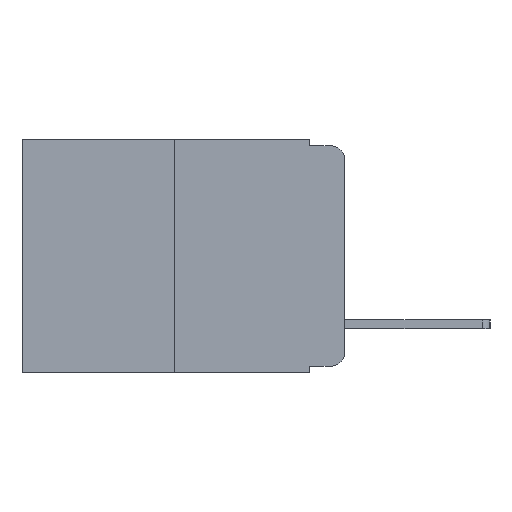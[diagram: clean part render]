
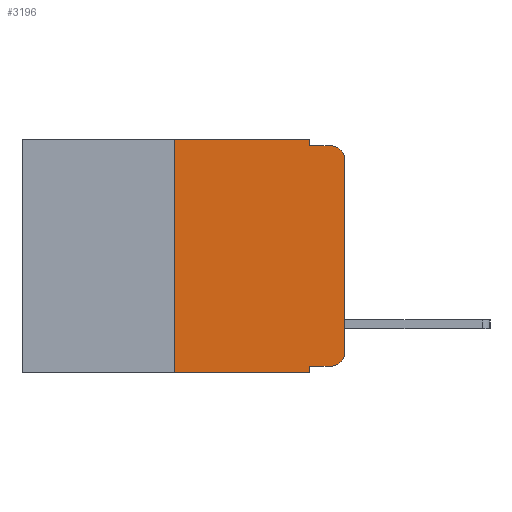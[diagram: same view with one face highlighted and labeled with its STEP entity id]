
A CAD part, left-side view. The second image highlights one B-rep face of the part: STEP entity #3196.
In plain terms, the highlighted planar face has unit normal (-1, 0, 0).
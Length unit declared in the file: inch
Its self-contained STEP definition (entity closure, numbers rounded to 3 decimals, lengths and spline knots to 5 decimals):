
#322 = EDGE_CURVE ( 'NONE', #18513, #15557, #9251, .T. ) ;
#994 = DIRECTION ( 'NONE',  ( 0., 0., 1. ) ) ;
#1172 = LINE ( 'NONE', #19652, #9362 ) ;
#1201 = ORIENTED_EDGE ( 'NONE', *, *, #19016, .F. ) ;
#1888 = DIRECTION ( 'NONE',  ( -1., 0., 0. ) ) ;
#2689 = CARTESIAN_POINT ( 'NONE',  ( 0., 0.051, -0.01 ) ) ;
#3196 = ADVANCED_FACE ( 'NONE', ( #18753 ), #17368, .F. ) ;
#3283 = ORIENTED_EDGE ( 'NONE', *, *, #15947, .F. ) ;
#3398 = VECTOR ( 'NONE', #13719, 39.37008 ) ;
#3613 = VECTOR ( 'NONE', #11609, 39.37008 ) ;
#3761 = VERTEX_POINT ( 'NONE', #12623 ) ;
#4547 = VERTEX_POINT ( 'NONE', #5112 ) ;
#4727 = LINE ( 'NONE', #5884, #12788 ) ;
#4770 = DIRECTION ( 'NONE',  ( 0., -1., 0. ) ) ;
#4900 = VERTEX_POINT ( 'NONE', #15831 ) ;
#5112 = CARTESIAN_POINT ( 'NONE',  ( 0., 0.25, -0.343 ) ) ;
#5862 = DIRECTION ( 'NONE',  ( 0., 0., -1. ) ) ;
#5884 = CARTESIAN_POINT ( 'NONE',  ( 0., 0., 0. ) ) ;
#6059 = CARTESIAN_POINT ( 'NONE',  ( 0., 0., -0.03 ) ) ;
#6288 = AXIS2_PLACEMENT_3D ( 'NONE', #11614, #1888, #13182 ) ;
#6341 = ORIENTED_EDGE ( 'NONE', *, *, #16486, .F. ) ;
#6467 = VERTEX_POINT ( 'NONE', #6059 ) ;
#6579 = CIRCLE ( 'NONE', #6288, 0.02 ) ;
#7234 = EDGE_CURVE ( 'NONE', #6467, #20227, #6579, .T. ) ;
#7325 = CARTESIAN_POINT ( 'NONE',  ( 0., 0.02, -0.313 ) ) ;
#7395 = EDGE_CURVE ( 'NONE', #20671, #7611, #10112, .T. ) ;
#7611 = VERTEX_POINT ( 'NONE', #8012 ) ;
#7755 = LINE ( 'NONE', #10516, #3398 ) ;
#7874 = DIRECTION ( 'NONE',  ( 1., 0., 0. ) ) ;
#8012 = CARTESIAN_POINT ( 'NONE',  ( 0., 0., -0.313 ) ) ;
#8069 = CARTESIAN_POINT ( 'NONE',  ( 0., 0.051, -0.333 ) ) ;
#8152 = ORIENTED_EDGE ( 'NONE', *, *, #10626, .T. ) ;
#8194 = EDGE_CURVE ( 'NONE', #4547, #3761, #9569, .T. ) ;
#8462 = LINE ( 'NONE', #9990, #3613 ) ;
#8744 = VECTOR ( 'NONE', #5862, 39.37008 ) ;
#8929 = DIRECTION ( 'NONE',  ( 0., 0., -1. ) ) ;
#9251 = LINE ( 'NONE', #17713, #8744 ) ;
#9362 = VECTOR ( 'NONE', #13468, 39.37008 ) ;
#9569 = LINE ( 'NONE', #17538, #17484 ) ;
#9679 = DIRECTION ( 'NONE',  ( 0., -1., 0. ) ) ;
#9990 = CARTESIAN_POINT ( 'NONE',  ( 0., 0.051, 0. ) ) ;
#10112 = CIRCLE ( 'NONE', #16995, 0.02 ) ;
#10162 = DIRECTION ( 'NONE',  ( 0., -1., 0. ) ) ;
#10207 = EDGE_LOOP ( 'NONE', ( #18019, #14394, #6341, #19964, #13643, #1201, #10905, #3283, #8152, #20697 ) ) ;
#10516 = CARTESIAN_POINT ( 'NONE',  ( 0., 0.473, 0. ) ) ;
#10626 = EDGE_CURVE ( 'NONE', #14865, #20671, #11202, .T. ) ;
#10905 = ORIENTED_EDGE ( 'NONE', *, *, #8194, .T. ) ;
#11202 = LINE ( 'NONE', #8069, #19018 ) ;
#11209 = VECTOR ( 'NONE', #10162, 39.37008 ) ;
#11609 = DIRECTION ( 'NONE',  ( 0., 0., -1. ) ) ;
#11614 = CARTESIAN_POINT ( 'NONE',  ( 0., 0.02, -0.03 ) ) ;
#12084 = EDGE_CURVE ( 'NONE', #4900, #18513, #7755, .T. ) ;
#12135 = CARTESIAN_POINT ( 'NONE',  ( 0., 0.051, -0.333 ) ) ;
#12215 = LINE ( 'NONE', #13364, #11209 ) ;
#12256 = CARTESIAN_POINT ( 'NONE',  ( 0., 0.051, 0. ) ) ;
#12623 = CARTESIAN_POINT ( 'NONE',  ( 0., 0.051, -0.343 ) ) ;
#12788 = VECTOR ( 'NONE', #994, 39.37008 ) ;
#13182 = DIRECTION ( 'NONE',  ( 0., 0., -1. ) ) ;
#13364 = CARTESIAN_POINT ( 'NONE',  ( 0., 0.051, -0.01 ) ) ;
#13468 = DIRECTION ( 'NONE',  ( 0., 0., 1. ) ) ;
#13643 = ORIENTED_EDGE ( 'NONE', *, *, #12084, .F. ) ;
#13719 = DIRECTION ( 'NONE',  ( 0., -1., 0. ) ) ;
#14394 = ORIENTED_EDGE ( 'NONE', *, *, #7234, .T. ) ;
#14865 = VERTEX_POINT ( 'NONE', #12135 ) ;
#15509 = CARTESIAN_POINT ( 'NONE',  ( 0., 0.02, -0.333 ) ) ;
#15557 = VERTEX_POINT ( 'NONE', #2689 ) ;
#15831 = CARTESIAN_POINT ( 'NONE',  ( 0., 0.25, 0. ) ) ;
#15947 = EDGE_CURVE ( 'NONE', #14865, #3761, #8462, .T. ) ;
#16486 = EDGE_CURVE ( 'NONE', #15557, #20227, #12215, .T. ) ;
#16995 = AXIS2_PLACEMENT_3D ( 'NONE', #7325, #18377, #8929 ) ;
#17368 = PLANE ( 'NONE',  #17789 ) ;
#17484 = VECTOR ( 'NONE', #4770, 39.37008 ) ;
#17538 = CARTESIAN_POINT ( 'NONE',  ( 0., 0.473, -0.343 ) ) ;
#17664 = CARTESIAN_POINT ( 'NONE',  ( 0., 0.02, -0.01 ) ) ;
#17713 = CARTESIAN_POINT ( 'NONE',  ( 0., 0.051, 0. ) ) ;
#17789 = AXIS2_PLACEMENT_3D ( 'NONE', #20415, #7874, #18898 ) ;
#18019 = ORIENTED_EDGE ( 'NONE', *, *, #20690, .T. ) ;
#18377 = DIRECTION ( 'NONE',  ( -1., 0., 0. ) ) ;
#18513 = VERTEX_POINT ( 'NONE', #12256 ) ;
#18753 = FACE_OUTER_BOUND ( 'NONE', #10207, .T. ) ;
#18898 = DIRECTION ( 'NONE',  ( 0., 0., -1. ) ) ;
#19016 = EDGE_CURVE ( 'NONE', #4547, #4900, #1172, .T. ) ;
#19018 = VECTOR ( 'NONE', #9679, 39.37008 ) ;
#19652 = CARTESIAN_POINT ( 'NONE',  ( 0., 0.25, 0. ) ) ;
#19964 = ORIENTED_EDGE ( 'NONE', *, *, #322, .F. ) ;
#20227 = VERTEX_POINT ( 'NONE', #17664 ) ;
#20415 = CARTESIAN_POINT ( 'NONE',  ( 0., 0.473, 0. ) ) ;
#20671 = VERTEX_POINT ( 'NONE', #15509 ) ;
#20690 = EDGE_CURVE ( 'NONE', #7611, #6467, #4727, .T. ) ;
#20697 = ORIENTED_EDGE ( 'NONE', *, *, #7395, .T. ) ;
